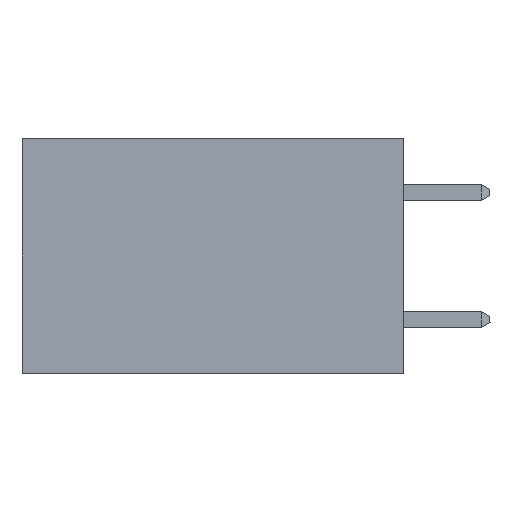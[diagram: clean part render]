
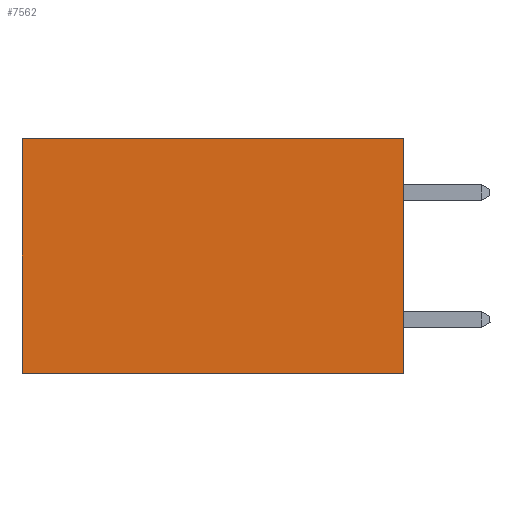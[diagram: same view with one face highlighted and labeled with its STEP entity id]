
A CAD part, left-side view. The second image highlights one B-rep face of the part: STEP entity #7562.
In plain terms, the highlighted planar face has unit normal (-1, 0, 0).
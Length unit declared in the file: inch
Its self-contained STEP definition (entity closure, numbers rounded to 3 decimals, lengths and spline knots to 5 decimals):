
#457 = CARTESIAN_POINT ( 'NONE',  ( 0.2875, 0., 0. ) ) ;
#729 = EDGE_LOOP ( 'NONE', ( #18698, #926, #20643, #9589 ) ) ;
#926 = ORIENTED_EDGE ( 'NONE', *, *, #2255, .F. ) ;
#1013 = CARTESIAN_POINT ( 'NONE',  ( 0.2875, 0., -0.37 ) ) ;
#1179 = VECTOR ( 'NONE', #12355, 39.37008 ) ;
#2169 = EDGE_CURVE ( 'NONE', #11347, #15783, #18126, .T. ) ;
#2255 = EDGE_CURVE ( 'NONE', #15783, #11084, #6284, .T. ) ;
#4189 = CARTESIAN_POINT ( 'NONE',  ( 0.2875, 0., 0. ) ) ;
#4731 = CARTESIAN_POINT ( 'NONE',  ( 0.2875, 0.6, 0. ) ) ;
#5222 = EDGE_CURVE ( 'NONE', #11347, #18008, #12201, .T. ) ;
#5658 = CARTESIAN_POINT ( 'NONE',  ( 0.2875, 0., 0. ) ) ;
#5732 = DIRECTION ( 'NONE',  ( 0., 0., -1. ) ) ;
#6016 = CARTESIAN_POINT ( 'NONE',  ( 0.2875, 0., 0. ) ) ;
#6284 = LINE ( 'NONE', #1013, #1179 ) ;
#7562 = ADVANCED_FACE ( 'NONE', ( #15273 ), #19974, .F. ) ;
#7666 = EDGE_CURVE ( 'NONE', #18008, #11084, #10969, .T. ) ;
#8927 = VECTOR ( 'NONE', #15243, 39.37008 ) ;
#9132 = CARTESIAN_POINT ( 'NONE',  ( 0.2875, 0., -0.37 ) ) ;
#9315 = AXIS2_PLACEMENT_3D ( 'NONE', #457, #18293, #10226 ) ;
#9589 = ORIENTED_EDGE ( 'NONE', *, *, #5222, .T. ) ;
#10226 = DIRECTION ( 'NONE',  ( 0., 0., -1. ) ) ;
#10969 = LINE ( 'NONE', #16931, #20653 ) ;
#11084 = VERTEX_POINT ( 'NONE', #18972 ) ;
#11347 = VERTEX_POINT ( 'NONE', #5658 ) ;
#12201 = LINE ( 'NONE', #4189, #8927 ) ;
#12355 = DIRECTION ( 'NONE',  ( 0., 1., 0. ) ) ;
#13082 = VECTOR ( 'NONE', #20609, 39.37008 ) ;
#15243 = DIRECTION ( 'NONE',  ( 0., 1., 0. ) ) ;
#15273 = FACE_OUTER_BOUND ( 'NONE', #729, .T. ) ;
#15783 = VERTEX_POINT ( 'NONE', #9132 ) ;
#16931 = CARTESIAN_POINT ( 'NONE',  ( 0.2875, 0.6, 0. ) ) ;
#18008 = VERTEX_POINT ( 'NONE', #4731 ) ;
#18126 = LINE ( 'NONE', #6016, #13082 ) ;
#18293 = DIRECTION ( 'NONE',  ( 1., 0., 0. ) ) ;
#18698 = ORIENTED_EDGE ( 'NONE', *, *, #7666, .T. ) ;
#18972 = CARTESIAN_POINT ( 'NONE',  ( 0.2875, 0.6, -0.37 ) ) ;
#19974 = PLANE ( 'NONE',  #9315 ) ;
#20609 = DIRECTION ( 'NONE',  ( 0., 0., -1. ) ) ;
#20643 = ORIENTED_EDGE ( 'NONE', *, *, #2169, .F. ) ;
#20653 = VECTOR ( 'NONE', #5732, 39.37008 ) ;
